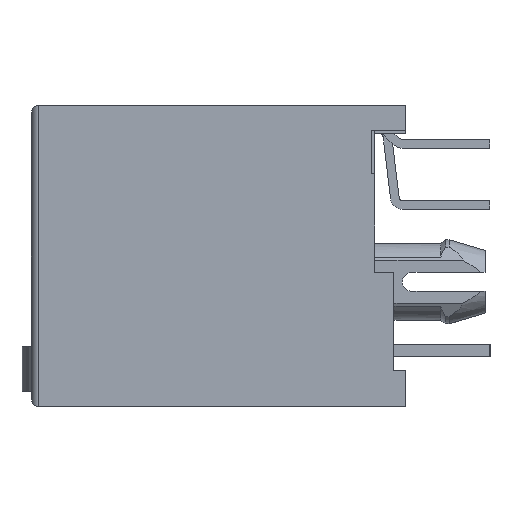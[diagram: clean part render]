
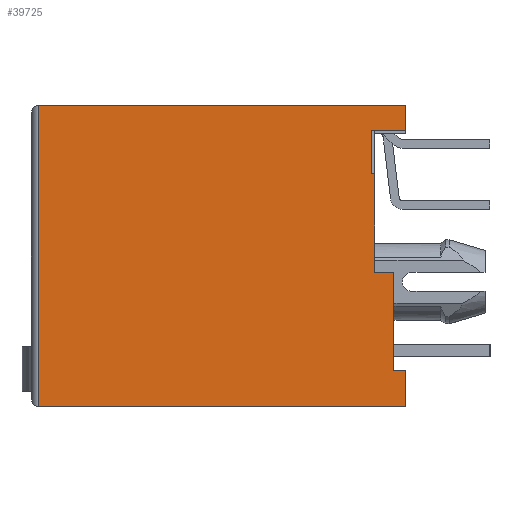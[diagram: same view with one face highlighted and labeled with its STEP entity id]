
A CAD part, left-side view. The second image highlights one B-rep face of the part: STEP entity #39725.
In plain terms, the highlighted planar face has unit normal (-1, 0, 0).
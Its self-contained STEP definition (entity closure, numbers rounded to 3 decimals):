
#394 = CARTESIAN_POINT ( 'NONE',  ( -31.5, -6.35, 3.45 ) ) ;
#553 = EDGE_CURVE ( 'NONE', #3208, #37782, #64171, .T. ) ;
#1446 = CARTESIAN_POINT ( 'NONE',  ( -31.5, -7.3, -4.75 ) ) ;
#3208 = VERTEX_POINT ( 'NONE', #54501 ) ;
#4085 = ORIENTED_EDGE ( 'NONE', *, *, #56124, .F. ) ;
#4800 = CARTESIAN_POINT ( 'NONE',  ( -31.5, -7.8, 5.95 ) ) ;
#4907 = CARTESIAN_POINT ( 'NONE',  ( -31.5, -7.8, -4.75 ) ) ;
#4960 = ORIENTED_EDGE ( 'NONE', *, *, #18181, .F. ) ;
#6356 = CARTESIAN_POINT ( 'NONE',  ( -31.5, -6.35, 4.65 ) ) ;
#6614 = EDGE_CURVE ( 'NONE', #24937, #12856, #43845, .T. ) ;
#7146 = EDGE_CURVE ( 'NONE', #19306, #26618, #45562, .T. ) ;
#7701 = CARTESIAN_POINT ( 'NONE',  ( -31.5, -7.467, -4.75 ) ) ;
#8012 = VERTEX_POINT ( 'NONE', #62502 ) ;
#9055 = FACE_OUTER_BOUND ( 'NONE', #16598, .T. ) ;
#9295 = B_SPLINE_CURVE_WITH_KNOTS ( 'NONE', 3,
 ( #20573, #21976, #31784, #59078 ),
 .UNSPECIFIED., .F., .F.,
 ( 4, 4 ),
 ( 0., 1. ),
 .UNSPECIFIED. ) ;
#9522 = B_SPLINE_CURVE_WITH_KNOTS ( 'NONE', 3,
 ( #65909, #25288, #56801, #25959 ),
 .UNSPECIFIED., .F., .F.,
 ( 4, 4 ),
 ( 0., 1. ),
 .UNSPECIFIED. ) ;
#10110 = CARTESIAN_POINT ( 'NONE',  ( -31.5, -7.8, -6.25 ) ) ;
#10374 = ORIENTED_EDGE ( 'NONE', *, *, #553, .F. ) ;
#10566 = ORIENTED_EDGE ( 'NONE', *, *, #32574, .F. ) ;
#10839 = CARTESIAN_POINT ( 'NONE',  ( -31.5, -6.5, 3.45 ) ) ;
#11361 = CARTESIAN_POINT ( 'NONE',  ( -31.5, -2.7, 6.3 ) ) ;
#11514 = CARTESIAN_POINT ( 'NONE',  ( -31.5, -6.4, 3.45 ) ) ;
#12856 = VERTEX_POINT ( 'NONE', #25228 ) ;
#14454 = CARTESIAN_POINT ( 'NONE',  ( -31.5, -7.8, -6.25 ) ) ;
#14813 = CARTESIAN_POINT ( 'NONE',  ( -31.5, 7.5, -2.067 ) ) ;
#14833 = EDGE_CURVE ( 'NONE', #54178, #19306, #38506, .T. ) ;
#15211 = CARTESIAN_POINT ( 'NONE',  ( -31.5, -6.35, 3.45 ) ) ;
#15310 = VERTEX_POINT ( 'NONE', #1446 ) ;
#15386 = CARTESIAN_POINT ( 'NONE',  ( -31.5, -6.45, 3.45 ) ) ;
#15936 = CARTESIAN_POINT ( 'NONE',  ( -31.5, -7.8, 6.3 ) ) ;
#16598 = EDGE_LOOP ( 'NONE', ( #10374, #38890, #10566, #27738, #4960, #36988, #29066, #4085, #63234, #47558, #47077, #31759 ) ) ;
#16977 = EDGE_CURVE ( 'NONE', #54178, #8012, #20467, .T. ) ;
#17686 = EDGE_CURVE ( 'NONE', #37782, #26618, #9522, .T. ) ;
#17830 = CARTESIAN_POINT ( 'NONE',  ( -31.5, -7.033, -0.65 ) ) ;
#18181 = EDGE_CURVE ( 'NONE', #60070, #24937, #38806, .T. ) ;
#18536 = CARTESIAN_POINT ( 'NONE',  ( -31.5, -6.767, -0.65 ) ) ;
#19194 = B_SPLINE_CURVE_WITH_KNOTS ( 'NONE', 3,
 ( #63369, #11514, #15386, #10839 ),
 .UNSPECIFIED., .F., .F.,
 ( 4, 4 ),
 ( 0., 1. ),
 .UNSPECIFIED. ) ;
#19306 = VERTEX_POINT ( 'NONE', #34195 ) ;
#19890 = DIRECTION ( 'NONE',  ( 0., 0., 1. ) ) ;
#20467 = B_SPLINE_CURVE_WITH_KNOTS ( 'NONE', 3,
 ( #15936, #4800, #68472, #20508 ),
 .UNSPECIFIED., .F., .F.,
 ( 4, 4 ),
 ( 0., 1. ),
 .UNSPECIFIED. ) ;
#20508 = CARTESIAN_POINT ( 'NONE',  ( -31.5, -7.8, 5.25 ) ) ;
#20573 = CARTESIAN_POINT ( 'NONE',  ( -31.5, -7.3, -0.65 ) ) ;
#21042 = CARTESIAN_POINT ( 'NONE',  ( -31.5, -7.8, 5.25 ) ) ;
#21829 = EDGE_CURVE ( 'NONE', #15310, #3208, #32385, .T. ) ;
#21976 = CARTESIAN_POINT ( 'NONE',  ( -31.5, -7.3, -2.017 ) ) ;
#22346 = CARTESIAN_POINT ( 'NONE',  ( -31.5, -7.317, 5.25 ) ) ;
#22547 = VERTEX_POINT ( 'NONE', #15211 ) ;
#23189 = VERTEX_POINT ( 'NONE', #56666 ) ;
#24937 = VERTEX_POINT ( 'NONE', #54794 ) ;
#25206 = CARTESIAN_POINT ( 'NONE',  ( -31.5, -7.8, -5.25 ) ) ;
#25228 = CARTESIAN_POINT ( 'NONE',  ( -31.5, -7.3, -0.65 ) ) ;
#25288 = CARTESIAN_POINT ( 'NONE',  ( -31.5, -2.7, -6.25 ) ) ;
#25959 = CARTESIAN_POINT ( 'NONE',  ( -31.5, 7.5, -6.25 ) ) ;
#26203 = DIRECTION ( 'NONE',  ( 1., 0., 0. ) ) ;
#26618 = VERTEX_POINT ( 'NONE', #55803 ) ;
#27623 = CARTESIAN_POINT ( 'NONE',  ( -31.5, -6.5, 2.083 ) ) ;
#27738 = ORIENTED_EDGE ( 'NONE', *, *, #6614, .F. ) ;
#28380 = AXIS2_PLACEMENT_3D ( 'NONE', #40936, #26203, #19890 ) ;
#29066 = ORIENTED_EDGE ( 'NONE', *, *, #58932, .F. ) ;
#31292 = CARTESIAN_POINT ( 'NONE',  ( -31.5, 7.5, 2.117 ) ) ;
#31759 = ORIENTED_EDGE ( 'NONE', *, *, #17686, .F. ) ;
#31784 = CARTESIAN_POINT ( 'NONE',  ( -31.5, -7.3, -3.383 ) ) ;
#32043 = CARTESIAN_POINT ( 'NONE',  ( -31.5, -7.8, 6.3 ) ) ;
#32219 = CARTESIAN_POINT ( 'NONE',  ( -31.5, -6.35, 4.05 ) ) ;
#32385 = B_SPLINE_CURVE_WITH_KNOTS ( 'NONE', 3,
 ( #62293, #7701, #40589, #67534 ),
 .UNSPECIFIED., .F., .F.,
 ( 4, 4 ),
 ( 0., 1. ),
 .UNSPECIFIED. ) ;
#32574 = EDGE_CURVE ( 'NONE', #12856, #15310, #9295, .T. ) ;
#33037 = EDGE_CURVE ( 'NONE', #22547, #60070, #19194, .T. ) ;
#34195 = CARTESIAN_POINT ( 'NONE',  ( -31.5, 7.5, 6.3 ) ) ;
#35576 = CARTESIAN_POINT ( 'NONE',  ( -31.5, -7.8, 6.3 ) ) ;
#35754 = B_SPLINE_CURVE_WITH_KNOTS ( 'NONE', 3,
 ( #21042, #22346, #42383, #59444 ),
 .UNSPECIFIED., .F., .F.,
 ( 4, 4 ),
 ( 0., 1. ),
 .UNSPECIFIED. ) ;
#36988 = ORIENTED_EDGE ( 'NONE', *, *, #33037, .F. ) ;
#37782 = VERTEX_POINT ( 'NONE', #14454 ) ;
#37827 = CARTESIAN_POINT ( 'NONE',  ( -31.5, -6.5, 3.45 ) ) ;
#38456 = CARTESIAN_POINT ( 'NONE',  ( -31.5, -6.5, -0.65 ) ) ;
#38506 = B_SPLINE_CURVE_WITH_KNOTS ( 'NONE', 3,
 ( #32043, #11361, #48523, #64598 ),
 .UNSPECIFIED., .F., .F.,
 ( 4, 4 ),
 ( 0., 1. ),
 .UNSPECIFIED. ) ;
#38806 = B_SPLINE_CURVE_WITH_KNOTS ( 'NONE', 3,
 ( #59111, #27623, #42302, #38456 ),
 .UNSPECIFIED., .F., .F.,
 ( 4, 4 ),
 ( 0., 1. ),
 .UNSPECIFIED. ) ;
#38890 = ORIENTED_EDGE ( 'NONE', *, *, #21829, .F. ) ;
#39725 = ADVANCED_FACE ( 'NONE', ( #9055 ), #46872, .F. ) ;
#39916 = CARTESIAN_POINT ( 'NONE',  ( -31.5, -7.3, -0.65 ) ) ;
#40589 = CARTESIAN_POINT ( 'NONE',  ( -31.5, -7.633, -4.75 ) ) ;
#40936 = CARTESIAN_POINT ( 'NONE',  ( -31.5, 7.806, -6.501 ) ) ;
#41784 = CARTESIAN_POINT ( 'NONE',  ( -31.5, 7.5, -6.25 ) ) ;
#42302 = CARTESIAN_POINT ( 'NONE',  ( -31.5, -6.5, 0.717 ) ) ;
#42383 = CARTESIAN_POINT ( 'NONE',  ( -31.5, -6.833, 5.25 ) ) ;
#43845 = B_SPLINE_CURVE_WITH_KNOTS ( 'NONE', 3,
 ( #44796, #18536, #17830, #39916 ),
 .UNSPECIFIED., .F., .F.,
 ( 4, 4 ),
 ( 0., 1. ),
 .UNSPECIFIED. ) ;
#44796 = CARTESIAN_POINT ( 'NONE',  ( -31.5, -6.5, -0.65 ) ) ;
#45562 = B_SPLINE_CURVE_WITH_KNOTS ( 'NONE', 3,
 ( #47064, #31292, #14813, #41784 ),
 .UNSPECIFIED., .F., .F.,
 ( 4, 4 ),
 ( 0., 1. ),
 .UNSPECIFIED. ) ;
#46872 = PLANE ( 'NONE',  #28380 ) ;
#47064 = CARTESIAN_POINT ( 'NONE',  ( -31.5, 7.5, 6.3 ) ) ;
#47077 = ORIENTED_EDGE ( 'NONE', *, *, #7146, .T. ) ;
#47558 = ORIENTED_EDGE ( 'NONE', *, *, #14833, .T. ) ;
#48523 = CARTESIAN_POINT ( 'NONE',  ( -31.5, 2.4, 6.3 ) ) ;
#49389 = CARTESIAN_POINT ( 'NONE',  ( -31.5, -6.35, 5.25 ) ) ;
#54178 = VERTEX_POINT ( 'NONE', #35576 ) ;
#54501 = CARTESIAN_POINT ( 'NONE',  ( -31.5, -7.8, -4.75 ) ) ;
#54794 = CARTESIAN_POINT ( 'NONE',  ( -31.5, -6.5, -0.65 ) ) ;
#55803 = CARTESIAN_POINT ( 'NONE',  ( -31.5, 7.5, -6.25 ) ) ;
#56124 = EDGE_CURVE ( 'NONE', #8012, #23189, #35754, .T. ) ;
#56666 = CARTESIAN_POINT ( 'NONE',  ( -31.5, -6.35, 5.25 ) ) ;
#56801 = CARTESIAN_POINT ( 'NONE',  ( -31.5, 2.4, -6.25 ) ) ;
#58932 = EDGE_CURVE ( 'NONE', #23189, #22547, #64020, .T. ) ;
#59078 = CARTESIAN_POINT ( 'NONE',  ( -31.5, -7.3, -4.75 ) ) ;
#59111 = CARTESIAN_POINT ( 'NONE',  ( -31.5, -6.5, 3.45 ) ) ;
#59444 = CARTESIAN_POINT ( 'NONE',  ( -31.5, -6.35, 5.25 ) ) ;
#60070 = VERTEX_POINT ( 'NONE', #37827 ) ;
#62293 = CARTESIAN_POINT ( 'NONE',  ( -31.5, -7.3, -4.75 ) ) ;
#62502 = CARTESIAN_POINT ( 'NONE',  ( -31.5, -7.8, 5.25 ) ) ;
#62653 = CARTESIAN_POINT ( 'NONE',  ( -31.5, -7.8, -5.75 ) ) ;
#63234 = ORIENTED_EDGE ( 'NONE', *, *, #16977, .F. ) ;
#63369 = CARTESIAN_POINT ( 'NONE',  ( -31.5, -6.35, 3.45 ) ) ;
#64020 = B_SPLINE_CURVE_WITH_KNOTS ( 'NONE', 3,
 ( #49389, #6356, #32219, #394 ),
 .UNSPECIFIED., .F., .F.,
 ( 4, 4 ),
 ( 0., 1. ),
 .UNSPECIFIED. ) ;
#64171 = B_SPLINE_CURVE_WITH_KNOTS ( 'NONE', 3,
 ( #4907, #25206, #62653, #10110 ),
 .UNSPECIFIED., .F., .F.,
 ( 4, 4 ),
 ( 0., 1. ),
 .UNSPECIFIED. ) ;
#64598 = CARTESIAN_POINT ( 'NONE',  ( -31.5, 7.5, 6.3 ) ) ;
#65909 = CARTESIAN_POINT ( 'NONE',  ( -31.5, -7.8, -6.25 ) ) ;
#67534 = CARTESIAN_POINT ( 'NONE',  ( -31.5, -7.8, -4.75 ) ) ;
#68472 = CARTESIAN_POINT ( 'NONE',  ( -31.5, -7.8, 5.6 ) ) ;
